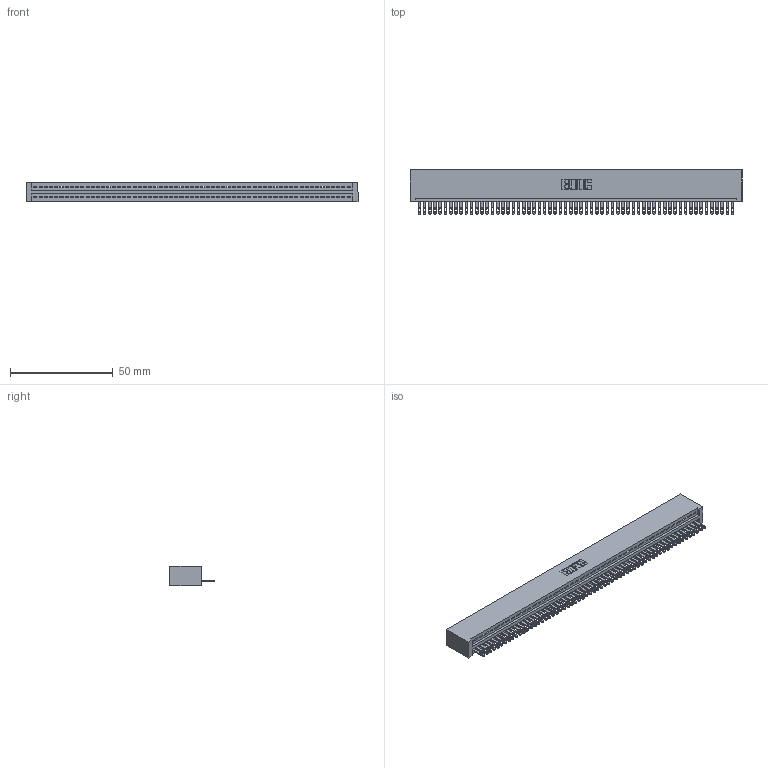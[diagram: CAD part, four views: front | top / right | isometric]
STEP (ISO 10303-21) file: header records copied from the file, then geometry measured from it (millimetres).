
FILE_DESCRIPTION (( 'STEP AP203' ), '1' );
FILE_NAME ('345-061-500-101.STEP', '2018-09-27T05:44:35', ( '' ), ( '' ), 'SwSTEP 2.0', 'SolidWorks 2016', '' );
FILE_SCHEMA (( 'CONFIG_CONTROL_DESIGN' ));
Length unit declared in the file: inch
Products named in the file (3): 345 Part_No Mounting Lugs; 345-061-500-101; 345-292-001_345-293-100
Assembly tree (62 placements, depth 2):
  345-061-500-101
    345 Part_No Mounting Lugs
    345-292-001_345-293-100  x61
Bounding box: 161.54 x 21.51 x 9.4 mm (x, y, z)
Volume: 16121.4 mm3; surface area: 22009.2 mm2
Topology: 62 solids, 62 shells, 3412 faces, 10565 edges, 7042 vertices
Faces by surface type: plane 2150, cylinder 1262
Entity records: 43005 total; most frequent: CARTESIAN_POINT 7455, ORIENTED_EDGE 7450, DIRECTION 6479, EDGE_CURVE 3725, LINE 3353, VECTOR 3353, VERTEX_POINT 2482, AXIS2_PLACEMENT_3D 1563
